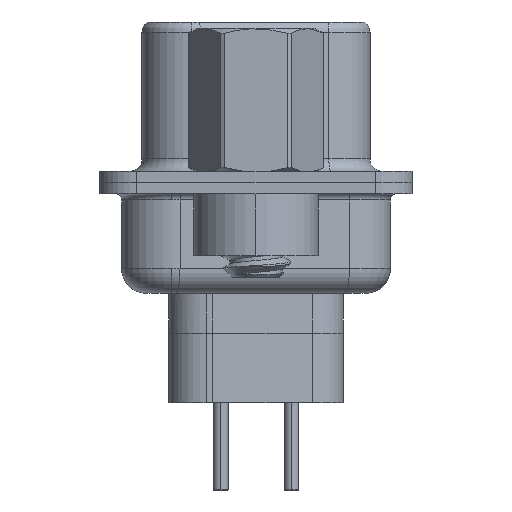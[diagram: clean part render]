
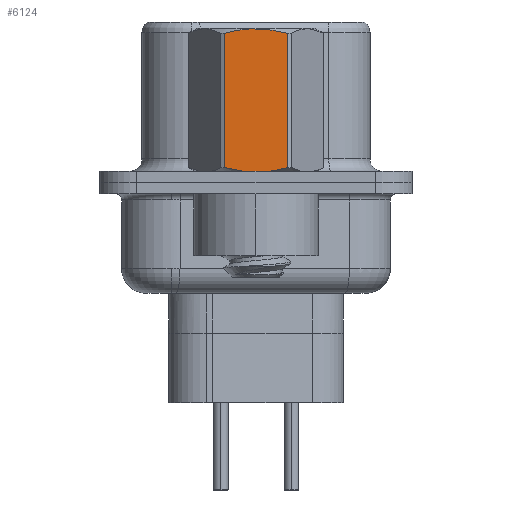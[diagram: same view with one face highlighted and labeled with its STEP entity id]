
A CAD part, left-side view. The second image highlights one B-rep face of the part: STEP entity #6124.
In plain terms, the highlighted planar face has unit normal (-1, 0, 0).
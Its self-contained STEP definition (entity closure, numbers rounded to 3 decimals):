
#1438 = CARTESIAN_POINT ( 'NONE',  ( -2.381, -0.432, 0.435 ) ) ;
#2253 = VERTEX_POINT ( 'NONE', #6439 ) ;
#2366 = CARTESIAN_POINT ( 'NONE',  ( -2.381, -1.273, 3.792 ) ) ;
#3017 = VECTOR ( 'NONE', #23426, 1000. ) ;
#3688 = CARTESIAN_POINT ( 'NONE',  ( -2.381, 1.273, 0.602 ) ) ;
#4240 = CARTESIAN_POINT ( 'NONE',  ( -2.381, -1.273, 0.602 ) ) ;
#4419 = LINE ( 'NONE', #2366, #21885 ) ;
#5583 = CARTESIAN_POINT ( 'NONE',  ( -2.381, 0.853, 0.499 ) ) ;
#6107 = PLANE ( 'NONE',  #25375 ) ;
#6124 = ADVANCED_FACE ( 'NONE', ( #27008 ), #6107, .T. ) ;
#6308 = CARTESIAN_POINT ( 'NONE',  ( -2.381, -1.273, 5.998 ) ) ;
#6439 = CARTESIAN_POINT ( 'NONE',  ( -2.381, -1.273, 5.998 ) ) ;
#7581 = VERTEX_POINT ( 'NONE', #4240 ) ;
#7614 = CARTESIAN_POINT ( 'NONE',  ( -2.381, 0.215, 0.418 ) ) ;
#7744 = CARTESIAN_POINT ( 'NONE',  ( -2.381, 1.375, -3.8 ) ) ;
#7981 = DIRECTION ( 'NONE',  ( 0., 0., 1. ) ) ;
#7988 = CARTESIAN_POINT ( 'NONE',  ( -2.381, 1.273, 5.998 ) ) ;
#8705 = CARTESIAN_POINT ( 'NONE',  ( -2.381, 1.273, 3.792 ) ) ;
#9052 = EDGE_CURVE ( 'NONE', #25696, #7581, #20378, .T. ) ;
#9945 = CARTESIAN_POINT ( 'NONE',  ( -2.381, 1.273, 0.602 ) ) ;
#10535 = CARTESIAN_POINT ( 'NONE',  ( -2.381, -0.215, 6.182 ) ) ;
#11111 = ORIENTED_EDGE ( 'NONE', *, *, #17767, .T. ) ;
#12258 = B_SPLINE_CURVE_WITH_KNOTS ( 'NONE', 3,
 ( #6308, #18817, #14659, #22539, #10535, #18540, #12587, #18678, #22674, #24745 ),
 .UNSPECIFIED., .F., .F.,
 ( 4, 2, 2, 2, 4 ),
 ( 0.001, 0.002, 0.002, 0.003, 0.004 ),
 .UNSPECIFIED. ) ;
#12587 = CARTESIAN_POINT ( 'NONE',  ( -2.381, 0.428, 6.165 ) ) ;
#13794 = CARTESIAN_POINT ( 'NONE',  ( -2.381, -1.273, 0.602 ) ) ;
#13923 = CARTESIAN_POINT ( 'NONE',  ( -2.381, 0.428, 0.435 ) ) ;
#14659 = CARTESIAN_POINT ( 'NONE',  ( -2.381, -0.858, 6.1 ) ) ;
#15979 = CARTESIAN_POINT ( 'NONE',  ( -2.381, -0.858, 0.5 ) ) ;
#16248 = DIRECTION ( 'NONE',  ( 0., -1., 0. ) ) ;
#17502 = LINE ( 'NONE', #8705, #3017 ) ;
#17767 = EDGE_CURVE ( 'NONE', #24859, #25696, #17502, .T. ) ;
#18540 = CARTESIAN_POINT ( 'NONE',  ( -2.381, 0.215, 6.182 ) ) ;
#18678 = CARTESIAN_POINT ( 'NONE',  ( -2.381, 0.853, 6.101 ) ) ;
#18817 = CARTESIAN_POINT ( 'NONE',  ( -2.381, -1.066, 6.054 ) ) ;
#20278 = CARTESIAN_POINT ( 'NONE',  ( -2.381, -1.066, 0.546 ) ) ;
#20291 = EDGE_CURVE ( 'NONE', #2253, #24859, #12258, .T. ) ;
#20378 = B_SPLINE_CURVE_WITH_KNOTS ( 'NONE', 3,
 ( #9945, #26887, #5583, #13923, #7614, #24404, #1438, #15979, #20278, #13794 ),
 .UNSPECIFIED., .F., .F.,
 ( 4, 2, 2, 2, 4 ),
 ( 0.003, 0.003, 0.004, 0.004, 0.005 ),
 .UNSPECIFIED. ) ;
#21885 = VECTOR ( 'NONE', #7981, 1000. ) ;
#22203 = ORIENTED_EDGE ( 'NONE', *, *, #9052, .T. ) ;
#22241 = ORIENTED_EDGE ( 'NONE', *, *, #24489, .T. ) ;
#22539 = CARTESIAN_POINT ( 'NONE',  ( -2.381, -0.432, 6.165 ) ) ;
#22674 = CARTESIAN_POINT ( 'NONE',  ( -2.381, 1.065, 6.054 ) ) ;
#23426 = DIRECTION ( 'NONE',  ( 0., 0., -1. ) ) ;
#23649 = ORIENTED_EDGE ( 'NONE', *, *, #20291, .T. ) ;
#24404 = CARTESIAN_POINT ( 'NONE',  ( -2.381, -0.215, 0.418 ) ) ;
#24489 = EDGE_CURVE ( 'NONE', #7581, #2253, #4419, .T. ) ;
#24533 = DIRECTION ( 'NONE',  ( -1., 0., 0. ) ) ;
#24591 = EDGE_LOOP ( 'NONE', ( #22203, #22241, #23649, #11111 ) ) ;
#24745 = CARTESIAN_POINT ( 'NONE',  ( -2.381, 1.273, 5.998 ) ) ;
#24859 = VERTEX_POINT ( 'NONE', #7988 ) ;
#25375 = AXIS2_PLACEMENT_3D ( 'NONE', #7744, #24533, #16248 ) ;
#25696 = VERTEX_POINT ( 'NONE', #3688 ) ;
#26887 = CARTESIAN_POINT ( 'NONE',  ( -2.381, 1.065, 0.546 ) ) ;
#27008 = FACE_OUTER_BOUND ( 'NONE', #24591, .T. ) ;
